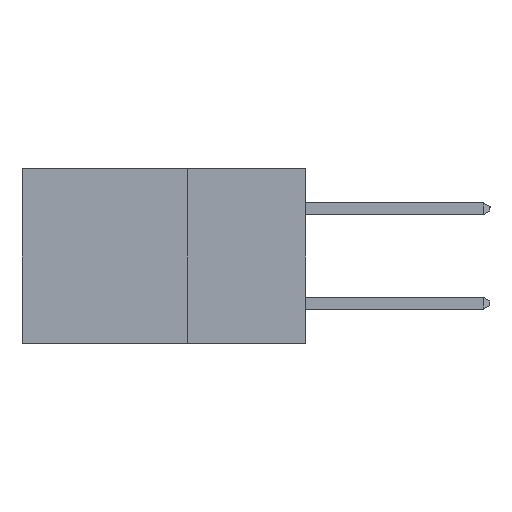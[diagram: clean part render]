
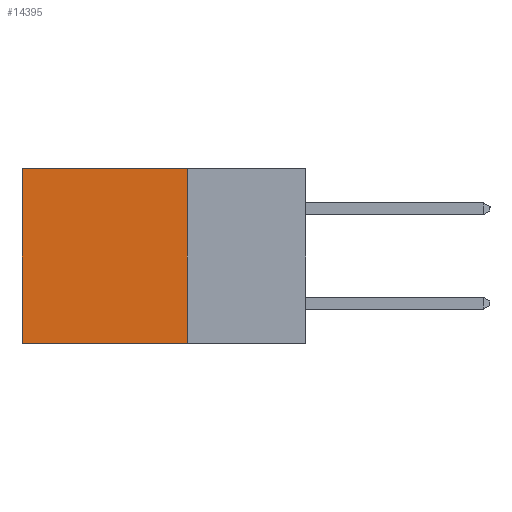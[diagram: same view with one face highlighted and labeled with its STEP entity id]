
A CAD part, left-side view. The second image highlights one B-rep face of the part: STEP entity #14395.
In plain terms, the highlighted planar face has unit normal (-1, 0, 0).
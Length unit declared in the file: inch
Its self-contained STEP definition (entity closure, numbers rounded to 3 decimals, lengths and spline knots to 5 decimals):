
#1199 = VERTEX_POINT ( 'NONE', #16224 ) ;
#1445 = VECTOR ( 'NONE', #6850, 39.37008 ) ;
#1920 = EDGE_LOOP ( 'NONE', ( #2885, #14410, #12564, #8656 ) ) ;
#2368 = VECTOR ( 'NONE', #6079, 39.37008 ) ;
#2566 = LINE ( 'NONE', #8009, #19027 ) ;
#2733 = DIRECTION ( 'NONE',  ( 1., 0., 0. ) ) ;
#2885 = ORIENTED_EDGE ( 'NONE', *, *, #15417, .T. ) ;
#3531 = VECTOR ( 'NONE', #13839, 39.37008 ) ;
#3829 = LINE ( 'NONE', #18868, #1445 ) ;
#4223 = VERTEX_POINT ( 'NONE', #5831 ) ;
#4453 = DIRECTION ( 'NONE',  ( 0., 1., 0. ) ) ;
#5162 = EDGE_CURVE ( 'NONE', #4223, #21434, #21413, .T. ) ;
#5831 = CARTESIAN_POINT ( 'NONE',  ( 0.2615, 0.25, 0. ) ) ;
#6079 = DIRECTION ( 'NONE',  ( 0., 0., -1. ) ) ;
#6089 = FACE_OUTER_BOUND ( 'NONE', #1920, .T. ) ;
#6348 = CARTESIAN_POINT ( 'NONE',  ( 0.2615, 0.6, 0. ) ) ;
#6487 = EDGE_CURVE ( 'NONE', #4223, #14082, #19122, .T. ) ;
#6850 = DIRECTION ( 'NONE',  ( 0., 0., -1. ) ) ;
#7727 = CARTESIAN_POINT ( 'NONE',  ( 0.2615, 0.25, -0.37 ) ) ;
#8009 = CARTESIAN_POINT ( 'NONE',  ( 0.2615, 0.25, -0.37 ) ) ;
#8656 = ORIENTED_EDGE ( 'NONE', *, *, #6487, .T. ) ;
#11228 = DIRECTION ( 'NONE',  ( 0., 0., -1. ) ) ;
#11384 = AXIS2_PLACEMENT_3D ( 'NONE', #7727, #2733, #11228 ) ;
#12467 = CARTESIAN_POINT ( 'NONE',  ( 0.2615, 0.25, -0.37 ) ) ;
#12564 = ORIENTED_EDGE ( 'NONE', *, *, #5162, .F. ) ;
#13839 = DIRECTION ( 'NONE',  ( 0., 1., 0. ) ) ;
#14082 = VERTEX_POINT ( 'NONE', #6348 ) ;
#14395 = ADVANCED_FACE ( 'NONE', ( #6089 ), #21105, .F. ) ;
#14410 = ORIENTED_EDGE ( 'NONE', *, *, #18907, .F. ) ;
#15417 = EDGE_CURVE ( 'NONE', #14082, #1199, #3829, .T. ) ;
#16224 = CARTESIAN_POINT ( 'NONE',  ( 0.2615, 0.6, -0.37 ) ) ;
#18868 = CARTESIAN_POINT ( 'NONE',  ( 0.2615, 0.6, -0.37 ) ) ;
#18898 = CARTESIAN_POINT ( 'NONE',  ( 0.2615, 0.25, 0. ) ) ;
#18907 = EDGE_CURVE ( 'NONE', #21434, #1199, #2566, .T. ) ;
#19027 = VECTOR ( 'NONE', #4453, 39.37008 ) ;
#19122 = LINE ( 'NONE', #18898, #3531 ) ;
#21105 = PLANE ( 'NONE',  #11384 ) ;
#21413 = LINE ( 'NONE', #12467, #2368 ) ;
#21434 = VERTEX_POINT ( 'NONE', #21638 ) ;
#21638 = CARTESIAN_POINT ( 'NONE',  ( 0.2615, 0.25, -0.37 ) ) ;
